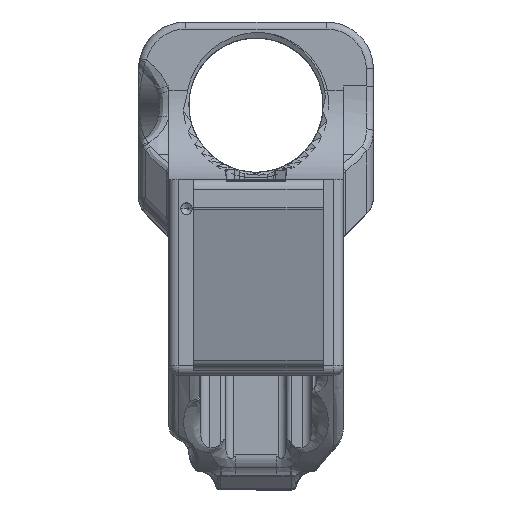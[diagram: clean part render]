
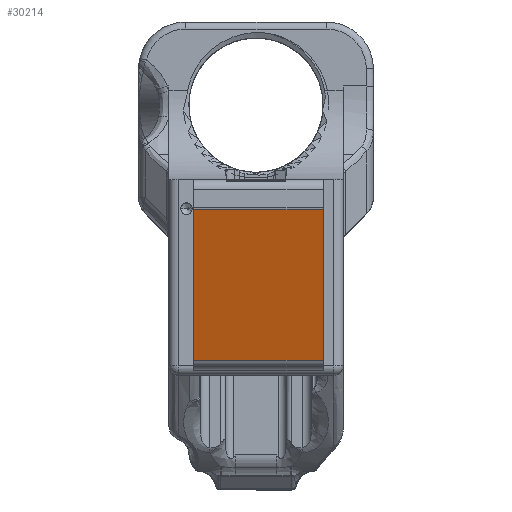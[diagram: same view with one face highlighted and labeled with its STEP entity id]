
A CAD part, top view. The second image highlights one B-rep face of the part: STEP entity #30214.
In plain terms, the highlighted planar face has unit normal (0, -0.287, 0.958).
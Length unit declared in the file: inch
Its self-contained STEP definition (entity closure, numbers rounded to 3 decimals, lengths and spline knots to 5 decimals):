
#149 = FACE_OUTER_BOUND ( 'NONE', #17068, .T. ) ;
#2500 = ORIENTED_EDGE ( 'NONE', *, *, #41659, .F. ) ;
#2664 = DIRECTION ( 'NONE',  ( -1., 0., 0. ) ) ;
#3690 = ORIENTED_EDGE ( 'NONE', *, *, #42095, .F. ) ;
#4362 = EDGE_CURVE ( 'NONE', #40056, #37508, #17896, .T. ) ;
#4739 = ORIENTED_EDGE ( 'NONE', *, *, #16257, .T. ) ;
#5027 = LINE ( 'NONE', #27281, #33987 ) ;
#6380 = DIRECTION ( 'NONE',  ( 0., -0.958, -0.287 ) ) ;
#8567 = AXIS2_PLACEMENT_3D ( 'NONE', #38193, #13911, #38339 ) ;
#10673 = VECTOR ( 'NONE', #32271, 39.37008 ) ;
#11379 = CARTESIAN_POINT ( 'NONE',  ( 2.03801, -0.17969, 3.20707 ) ) ;
#12860 = VERTEX_POINT ( 'NONE', #19189 ) ;
#13212 = CARTESIAN_POINT ( 'NONE',  ( 1.29347, 1.07844, 3.58419 ) ) ;
#13911 = DIRECTION ( 'NONE',  ( 0., 0.287, -0.958 ) ) ;
#13964 = VECTOR ( 'NONE', #44655, 39.37008 ) ;
#14326 = ORIENTED_EDGE ( 'NONE', *, *, #4362, .T. ) ;
#14899 = CARTESIAN_POINT ( 'NONE',  ( 0.20897, -0.17969, 3.20707 ) ) ;
#16257 = EDGE_CURVE ( 'NONE', #37508, #22813, #5027, .T. ) ;
#17068 = EDGE_LOOP ( 'NONE', ( #3690, #2500, #14326, #4739 ) ) ;
#17442 = CARTESIAN_POINT ( 'NONE',  ( 0.20897, 1.07844, 3.58419 ) ) ;
#17780 = LINE ( 'NONE', #11379, #10673 ) ;
#17896 = LINE ( 'NONE', #20045, #36480 ) ;
#19189 = CARTESIAN_POINT ( 'NONE',  ( 1.29347, -0.17969, 3.20707 ) ) ;
#20045 = CARTESIAN_POINT ( 'NONE',  ( 0.20897, 1.07844, 3.58419 ) ) ;
#22813 = VERTEX_POINT ( 'NONE', #14899 ) ;
#23219 = LINE ( 'NONE', #13212, #13964 ) ;
#27281 = CARTESIAN_POINT ( 'NONE',  ( 0.20897, -0.89688, 2.99209 ) ) ;
#30214 = ADVANCED_FACE ( 'NONE', ( #149 ), #34842, .F. ) ;
#32271 = DIRECTION ( 'NONE',  ( -1., 0., 0. ) ) ;
#33987 = VECTOR ( 'NONE', #6380, 39.37008 ) ;
#34842 = PLANE ( 'NONE',  #8567 ) ;
#36480 = VECTOR ( 'NONE', #2664, 39.37008 ) ;
#37508 = VERTEX_POINT ( 'NONE', #17442 ) ;
#38193 = CARTESIAN_POINT ( 'NONE',  ( 2.03801, -0.89688, 2.99209 ) ) ;
#38339 = DIRECTION ( 'NONE',  ( 0., 0.958, 0.287 ) ) ;
#40056 = VERTEX_POINT ( 'NONE', #42119 ) ;
#41659 = EDGE_CURVE ( 'NONE', #40056, #12860, #23219, .T. ) ;
#42095 = EDGE_CURVE ( 'NONE', #12860, #22813, #17780, .T. ) ;
#42119 = CARTESIAN_POINT ( 'NONE',  ( 1.29347, 1.07844, 3.58419 ) ) ;
#44655 = DIRECTION ( 'NONE',  ( 0., -0.958, -0.287 ) ) ;
